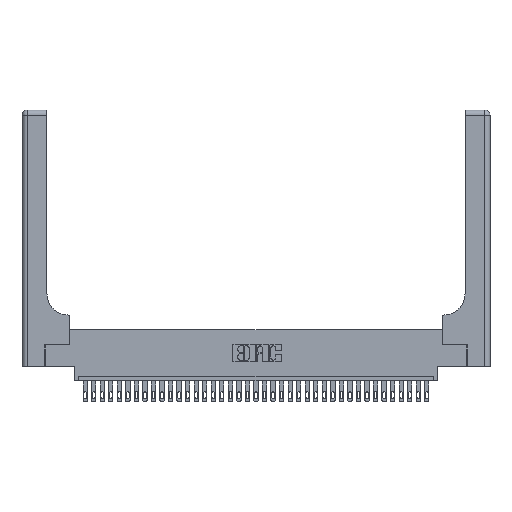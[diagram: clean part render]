
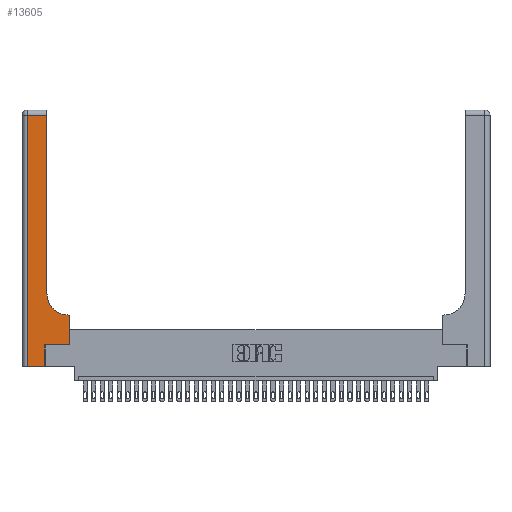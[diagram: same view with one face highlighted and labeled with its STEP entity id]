
A CAD part, top view. The second image highlights one B-rep face of the part: STEP entity #13605.
In plain terms, the highlighted planar face has unit normal (0, 0, 1).
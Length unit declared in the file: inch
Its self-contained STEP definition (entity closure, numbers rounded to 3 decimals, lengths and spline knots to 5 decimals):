
#290 = EDGE_CURVE ( 'NONE', #16641, #26768, #25634, .T. ) ;
#1425 = CARTESIAN_POINT ( 'NONE',  ( 0.5585, 0.6, 0.37 ) ) ;
#2422 = CARTESIAN_POINT ( 'NONE',  ( 0.269, 0.25, 0.37 ) ) ;
#2901 = ORIENTED_EDGE ( 'NONE', *, *, #290, .T. ) ;
#4393 = VECTOR ( 'NONE', #8873, 39.37008 ) ;
#5111 = DIRECTION ( 'NONE',  ( 0., 0., -1. ) ) ;
#5740 = AXIS2_PLACEMENT_3D ( 'NONE', #21909, #5111, #24916 ) ;
#6019 = ORIENTED_EDGE ( 'NONE', *, *, #33769, .T. ) ;
#6186 = CARTESIAN_POINT ( 'NONE',  ( 0.2915, 3., 0.37 ) ) ;
#6243 = LINE ( 'NONE', #6697, #34262 ) ;
#6419 = CARTESIAN_POINT ( 'NONE',  ( 0.2915, 0.6, 0.37 ) ) ;
#6697 = CARTESIAN_POINT ( 'NONE',  ( 0.5585, 0.25, 0.37 ) ) ;
#6966 = DIRECTION ( 'NONE',  ( 0., 1., 0. ) ) ;
#7096 = VECTOR ( 'NONE', #29529, 39.37008 ) ;
#7217 = VECTOR ( 'NONE', #21455, 39.37008 ) ;
#7406 = LINE ( 'NONE', #6419, #36260 ) ;
#8873 = DIRECTION ( 'NONE',  ( 0., 1., 0. ) ) ;
#9122 = FACE_OUTER_BOUND ( 'NONE', #29469, .T. ) ;
#9445 = CARTESIAN_POINT ( 'NONE',  ( 0.5415, 0.85, 0.37 ) ) ;
#11107 = VECTOR ( 'NONE', #24466, 39.37008 ) ;
#11159 = ORIENTED_EDGE ( 'NONE', *, *, #32694, .T. ) ;
#12435 = VERTEX_POINT ( 'NONE', #26517 ) ;
#12613 = LINE ( 'NONE', #31191, #25283 ) ;
#12978 = CARTESIAN_POINT ( 'NONE',  ( 0.06, 2.94, 0.37 ) ) ;
#13605 = ADVANCED_FACE ( 'NONE', ( #9122 ), #19083, .F. ) ;
#13641 = CARTESIAN_POINT ( 'NONE',  ( 0.269, 0., 0.37 ) ) ;
#14065 = ORIENTED_EDGE ( 'NONE', *, *, #16180, .T. ) ;
#14333 = ORIENTED_EDGE ( 'NONE', *, *, #16383, .T. ) ;
#14579 = DIRECTION ( 'NONE',  ( 1., 0., 0. ) ) ;
#14777 = CARTESIAN_POINT ( 'NONE',  ( 0.5585, 0.25, 0.37 ) ) ;
#16180 = EDGE_CURVE ( 'NONE', #31263, #32596, #30791, .T. ) ;
#16383 = EDGE_CURVE ( 'NONE', #22681, #22787, #6243, .T. ) ;
#16641 = VERTEX_POINT ( 'NONE', #30558 ) ;
#17530 = VERTEX_POINT ( 'NONE', #12978 ) ;
#17573 = DIRECTION ( 'NONE',  ( -1., 0., 0. ) ) ;
#17894 = VERTEX_POINT ( 'NONE', #29404 ) ;
#18436 = AXIS2_PLACEMENT_3D ( 'NONE', #9445, #31311, #14579 ) ;
#18727 = ORIENTED_EDGE ( 'NONE', *, *, #28023, .T. ) ;
#19083 = PLANE ( 'NONE',  #5740 ) ;
#19827 = CARTESIAN_POINT ( 'NONE',  ( 0.269, 0., 0.37 ) ) ;
#21455 = DIRECTION ( 'NONE',  ( 1., 0., 0. ) ) ;
#21612 = LINE ( 'NONE', #29280, #7096 ) ;
#21909 = CARTESIAN_POINT ( 'NONE',  ( 0., 3., 0.37 ) ) ;
#22381 = VECTOR ( 'NONE', #30352, 39.37008 ) ;
#22681 = VERTEX_POINT ( 'NONE', #14777 ) ;
#22787 = VERTEX_POINT ( 'NONE', #1425 ) ;
#22933 = EDGE_CURVE ( 'NONE', #12435, #22681, #33434, .T. ) ;
#23034 = ORIENTED_EDGE ( 'NONE', *, *, #22933, .T. ) ;
#24466 = DIRECTION ( 'NONE',  ( 1., 0., 0. ) ) ;
#24916 = DIRECTION ( 'NONE',  ( -1., 0., 0. ) ) ;
#24950 = CARTESIAN_POINT ( 'NONE',  ( 0.06, 0., 0.37 ) ) ;
#25283 = VECTOR ( 'NONE', #34006, 39.37008 ) ;
#25634 = CIRCLE ( 'NONE', #18436, 0.25 ) ;
#26517 = CARTESIAN_POINT ( 'NONE',  ( 0.269, 0.25, 0.37 ) ) ;
#26768 = VERTEX_POINT ( 'NONE', #33191 ) ;
#27359 = ORIENTED_EDGE ( 'NONE', *, *, #28721, .T. ) ;
#28023 = EDGE_CURVE ( 'NONE', #32596, #12435, #30204, .T. ) ;
#28721 = EDGE_CURVE ( 'NONE', #22787, #16641, #7406, .T. ) ;
#29280 = CARTESIAN_POINT ( 'NONE',  ( 0.06, 3., 0.37 ) ) ;
#29281 = LINE ( 'NONE', #6186, #4393 ) ;
#29352 = EDGE_CURVE ( 'NONE', #17894, #17530, #12613, .T. ) ;
#29404 = CARTESIAN_POINT ( 'NONE',  ( 0.2915, 2.94, 0.37 ) ) ;
#29469 = EDGE_LOOP ( 'NONE', ( #6019, #31462, #11159, #14065, #18727, #23034, #14333, #27359, #2901 ) ) ;
#29529 = DIRECTION ( 'NONE',  ( 0., -1., 0. ) ) ;
#30204 = LINE ( 'NONE', #13641, #22381 ) ;
#30352 = DIRECTION ( 'NONE',  ( 0., 1., 0. ) ) ;
#30558 = CARTESIAN_POINT ( 'NONE',  ( 0.5415, 0.6, 0.37 ) ) ;
#30791 = LINE ( 'NONE', #35447, #7217 ) ;
#31191 = CARTESIAN_POINT ( 'NONE',  ( 0., 2.94, 0.37 ) ) ;
#31263 = VERTEX_POINT ( 'NONE', #24950 ) ;
#31311 = DIRECTION ( 'NONE',  ( 0., 0., -1. ) ) ;
#31462 = ORIENTED_EDGE ( 'NONE', *, *, #29352, .T. ) ;
#32596 = VERTEX_POINT ( 'NONE', #19827 ) ;
#32694 = EDGE_CURVE ( 'NONE', #17530, #31263, #21612, .T. ) ;
#33191 = CARTESIAN_POINT ( 'NONE',  ( 0.2915, 0.85, 0.37 ) ) ;
#33434 = LINE ( 'NONE', #2422, #11107 ) ;
#33769 = EDGE_CURVE ( 'NONE', #26768, #17894, #29281, .T. ) ;
#34006 = DIRECTION ( 'NONE',  ( -1., 0., 0. ) ) ;
#34262 = VECTOR ( 'NONE', #6966, 39.37008 ) ;
#35447 = CARTESIAN_POINT ( 'NONE',  ( 0., 0., 0.37 ) ) ;
#36260 = VECTOR ( 'NONE', #17573, 39.37008 ) ;
